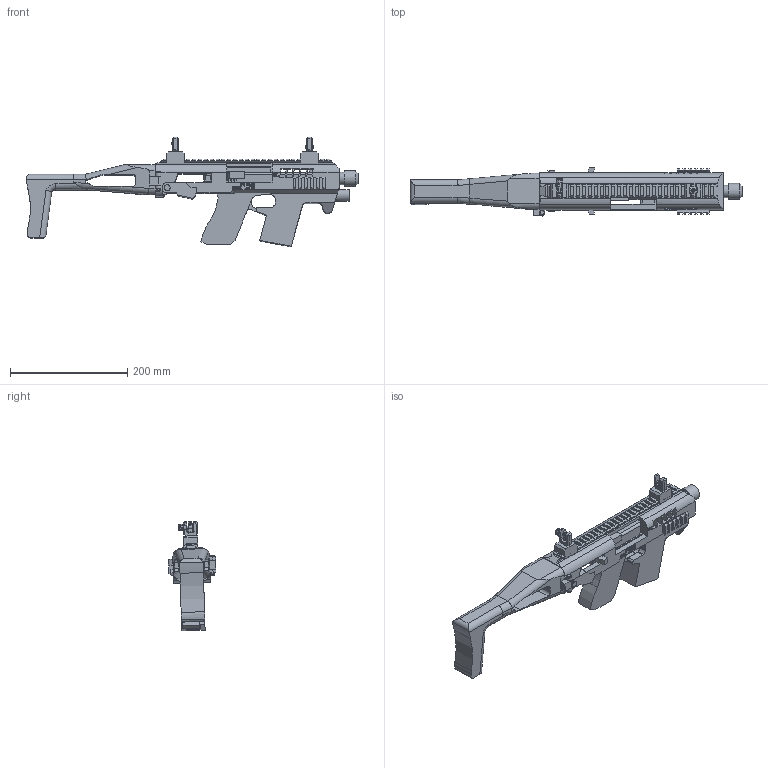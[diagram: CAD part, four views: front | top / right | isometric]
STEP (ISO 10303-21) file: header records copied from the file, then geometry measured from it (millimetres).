
FILE_DESCRIPTION(/* description */ ('Unknown'),/* implementation_level */ '2;1');
FILE_NAME(/* name */ 'Micro Roni + Glock 17',/* time_stamp */ '2018-12-18T17:33:29+02:00',/* author */ ('Unknown'),/* organization */ ('Unknown'),/* preprocessor_version */ 'ST-DEVELOPER v16.7',/* originating_system */ 'DEX',/* authorisation */ $);
FILE_SCHEMA (('AUTOMOTIVE_DESIGN {1 0 10303 214 3 1 1}'));
Length unit declared in the file: millimetre
Products named in the file (12): Micro Roni + Glock 17; Glock 17; Micro roni íàñàäêà; Micro roni 膰豵鵨; Micro roni ïðèêëàä; Micro roni 鳱歑攡; Micro roni øòèôò; Micro roni øòèôò1; Micro roni 瀔儗槶 1; Micro roni 瀔儗槶 2; Âèíò äëÿ øòèôòà; Âèíò äëÿ øòèôòà1
Assembly tree (11 placements, depth 2):
  Micro Roni + Glock 17
    Glock 17
    Micro roni íàñàäêà
    Micro roni 膰豵鵨
    Micro roni ïðèêëàä
    Micro roni 鳱歑攡
    Micro roni øòèôò
    Micro roni øòèôò1
    Micro roni 瀔儗槶 1
    Micro roni 瀔儗槶 2
    Âèíò äëÿ øòèôòà
    Âèíò äëÿ øòèôòà1
Bounding box: 567.51 x 82.02 x 187.65 mm (x, y, z)
Volume: 1496766.7 mm3; surface area: 285382.2 mm2
Topology: 11 solids, 11 shells, 1308 faces, 3732 edges, 2469 vertices
Faces by surface type: plane 1092, cylinder 198, torus 12, bspline 4, cone 2
Full cylindrical faces by diameter (mm): 1 x1, 2 x1, 4 x5, 4.134 x1, 5 x5, 5.917 x1, 6 x1, 7 x6, 9 x1, 10 x1, 11.5 x1, 14.5 x1, 15 x1, 20 x1, 21.237 x1, 27.237 x1
Entity records: 42608 total; most frequent: CARTESIAN_POINT 7802, ORIENTED_EDGE 7366, DIRECTION 6744, EDGE_CURVE 3683, LINE 3128, VECTOR 3128, VERTEX_POINT 2453, AXIS2_PLACEMENT_3D 1808
